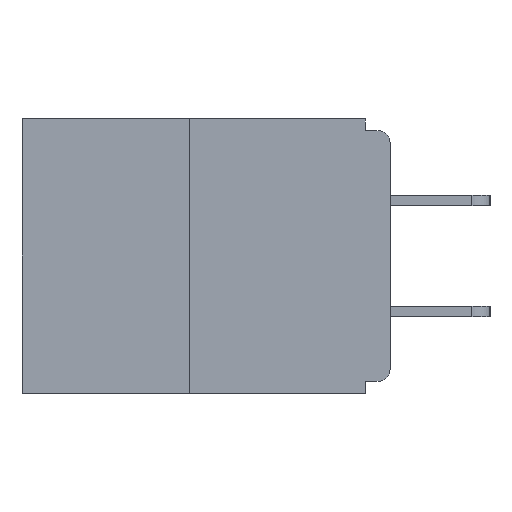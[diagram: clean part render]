
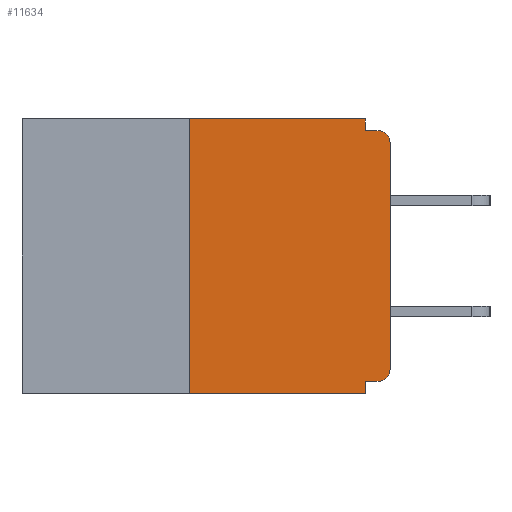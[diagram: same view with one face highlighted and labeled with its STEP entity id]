
A CAD part, left-side view. The second image highlights one B-rep face of the part: STEP entity #11634.
In plain terms, the highlighted planar face has unit normal (-1, 0, 0).
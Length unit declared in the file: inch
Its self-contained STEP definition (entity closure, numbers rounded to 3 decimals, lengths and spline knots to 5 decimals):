
#259 = DIRECTION ( 'NONE',  ( -1., 0., 0. ) ) ;
#296 = DIRECTION ( 'NONE',  ( 0., 0., -1. ) ) ;
#310 = DIRECTION ( 'NONE',  ( 0., 0., 1. ) ) ;
#486 = AXIS2_PLACEMENT_3D ( 'NONE', #3055, #259, #6879 ) ;
#506 = DIRECTION ( 'NONE',  ( 0., 0., -1. ) ) ;
#751 = CARTESIAN_POINT ( 'NONE',  ( 0., 0., -0.015 ) ) ;
#827 = LINE ( 'NONE', #751, #10610 ) ;
#847 = VECTOR ( 'NONE', #3934, 39.37008 ) ;
#923 = VERTEX_POINT ( 'NONE', #5600 ) ;
#1059 = LINE ( 'NONE', #4057, #7824 ) ;
#1091 = VERTEX_POINT ( 'NONE', #5325 ) ;
#1187 = ORIENTED_EDGE ( 'NONE', *, *, #7943, .T. ) ;
#1335 = CARTESIAN_POINT ( 'NONE',  ( 0., 0., -0.328 ) ) ;
#1851 = VECTOR ( 'NONE', #10932, 39.37008 ) ;
#1880 = EDGE_CURVE ( 'NONE', #6615, #6123, #10182, .T. ) ;
#1933 = ORIENTED_EDGE ( 'NONE', *, *, #2300, .F. ) ;
#2059 = CARTESIAN_POINT ( 'NONE',  ( 0., 0.031, -0.343 ) ) ;
#2085 = VERTEX_POINT ( 'NONE', #10942 ) ;
#2130 = DIRECTION ( 'NONE',  ( 1., 0., 0. ) ) ;
#2300 = EDGE_CURVE ( 'NONE', #6615, #12089, #1059, .T. ) ;
#2381 = CARTESIAN_POINT ( 'NONE',  ( 0., 0., -0.03 ) ) ;
#2758 = VERTEX_POINT ( 'NONE', #3836 ) ;
#2936 = EDGE_CURVE ( 'NONE', #10564, #5467, #3871, .T. ) ;
#3055 = CARTESIAN_POINT ( 'NONE',  ( 0., 0.015, -0.313 ) ) ;
#3077 = CARTESIAN_POINT ( 'NONE',  ( 0., 0.015, -0.015 ) ) ;
#3119 = DIRECTION ( 'NONE',  ( 0., 0., 1. ) ) ;
#3183 = VECTOR ( 'NONE', #9500, 39.37008 ) ;
#3238 = VECTOR ( 'NONE', #7019, 39.37008 ) ;
#3256 = LINE ( 'NONE', #8632, #6052 ) ;
#3456 = ORIENTED_EDGE ( 'NONE', *, *, #6091, .T. ) ;
#3460 = DIRECTION ( 'NONE',  ( 0., -1., 0. ) ) ;
#3487 = CARTESIAN_POINT ( 'NONE',  ( 0., 0.031, -0.343 ) ) ;
#3836 = CARTESIAN_POINT ( 'NONE',  ( 0., 0.015, -0.328 ) ) ;
#3871 = CIRCLE ( 'NONE', #6202, 0.015 ) ;
#3910 = LINE ( 'NONE', #6048, #1851 ) ;
#3934 = DIRECTION ( 'NONE',  ( 0., 0., -1. ) ) ;
#3982 = EDGE_LOOP ( 'NONE', ( #10138, #1933, #8150, #6756, #4250, #1187, #3456, #6971, #9232, #10843 ) ) ;
#4057 = CARTESIAN_POINT ( 'NONE',  ( 0., 0.25, 0. ) ) ;
#4250 = ORIENTED_EDGE ( 'NONE', *, *, #5422, .F. ) ;
#4521 = CARTESIAN_POINT ( 'NONE',  ( 0., 0., -0.313 ) ) ;
#4804 = FACE_OUTER_BOUND ( 'NONE', #3982, .T. ) ;
#4820 = VERTEX_POINT ( 'NONE', #4521 ) ;
#5325 = CARTESIAN_POINT ( 'NONE',  ( 0., 0.031, -0.328 ) ) ;
#5422 = EDGE_CURVE ( 'NONE', #2758, #1091, #8515, .T. ) ;
#5467 = VERTEX_POINT ( 'NONE', #3077 ) ;
#5532 = CIRCLE ( 'NONE', #486, 0.015 ) ;
#5577 = VECTOR ( 'NONE', #3119, 39.37008 ) ;
#5600 = CARTESIAN_POINT ( 'NONE',  ( 0., 0.031, 0. ) ) ;
#6048 = CARTESIAN_POINT ( 'NONE',  ( 0., 0.46, 0. ) ) ;
#6052 = VECTOR ( 'NONE', #296, 39.37008 ) ;
#6091 = EDGE_CURVE ( 'NONE', #4820, #10564, #7446, .T. ) ;
#6123 = VERTEX_POINT ( 'NONE', #3487 ) ;
#6202 = AXIS2_PLACEMENT_3D ( 'NONE', #8009, #10856, #506 ) ;
#6615 = VERTEX_POINT ( 'NONE', #7360 ) ;
#6756 = ORIENTED_EDGE ( 'NONE', *, *, #11001, .F. ) ;
#6879 = DIRECTION ( 'NONE',  ( 0., 0., -1. ) ) ;
#6907 = EDGE_CURVE ( 'NONE', #12089, #923, #3910, .T. ) ;
#6971 = ORIENTED_EDGE ( 'NONE', *, *, #2936, .T. ) ;
#7019 = DIRECTION ( 'NONE',  ( 0., 1., 0. ) ) ;
#7360 = CARTESIAN_POINT ( 'NONE',  ( 0., 0.25, -0.343 ) ) ;
#7446 = LINE ( 'NONE', #8784, #5577 ) ;
#7710 = PLANE ( 'NONE',  #10645 ) ;
#7824 = VECTOR ( 'NONE', #310, 39.37008 ) ;
#7943 = EDGE_CURVE ( 'NONE', #2758, #4820, #5532, .T. ) ;
#8009 = CARTESIAN_POINT ( 'NONE',  ( 0., 0.015, -0.03 ) ) ;
#8150 = ORIENTED_EDGE ( 'NONE', *, *, #1880, .T. ) ;
#8492 = CARTESIAN_POINT ( 'NONE',  ( 0., 0.46, -0.343 ) ) ;
#8515 = LINE ( 'NONE', #1335, #3238 ) ;
#8563 = EDGE_CURVE ( 'NONE', #923, #2085, #3256, .T. ) ;
#8632 = CARTESIAN_POINT ( 'NONE',  ( 0., 0.031, 0. ) ) ;
#8784 = CARTESIAN_POINT ( 'NONE',  ( 0., 0., 0. ) ) ;
#9232 = ORIENTED_EDGE ( 'NONE', *, *, #11909, .F. ) ;
#9500 = DIRECTION ( 'NONE',  ( 0., -1., 0. ) ) ;
#9917 = LINE ( 'NONE', #2059, #847 ) ;
#10138 = ORIENTED_EDGE ( 'NONE', *, *, #6907, .F. ) ;
#10182 = LINE ( 'NONE', #8492, #3183 ) ;
#10478 = DIRECTION ( 'NONE',  ( 0., 0., -1. ) ) ;
#10564 = VERTEX_POINT ( 'NONE', #2381 ) ;
#10610 = VECTOR ( 'NONE', #3460, 39.37008 ) ;
#10645 = AXIS2_PLACEMENT_3D ( 'NONE', #11593, #2130, #10478 ) ;
#10843 = ORIENTED_EDGE ( 'NONE', *, *, #8563, .F. ) ;
#10856 = DIRECTION ( 'NONE',  ( -1., 0., 0. ) ) ;
#10932 = DIRECTION ( 'NONE',  ( 0., -1., 0. ) ) ;
#10942 = CARTESIAN_POINT ( 'NONE',  ( 0., 0.031, -0.015 ) ) ;
#11001 = EDGE_CURVE ( 'NONE', #1091, #6123, #9917, .T. ) ;
#11379 = CARTESIAN_POINT ( 'NONE',  ( 0., 0.25, 0. ) ) ;
#11593 = CARTESIAN_POINT ( 'NONE',  ( 0., 0.46, 0. ) ) ;
#11634 = ADVANCED_FACE ( 'NONE', ( #4804 ), #7710, .F. ) ;
#11909 = EDGE_CURVE ( 'NONE', #2085, #5467, #827, .T. ) ;
#12089 = VERTEX_POINT ( 'NONE', #11379 ) ;
